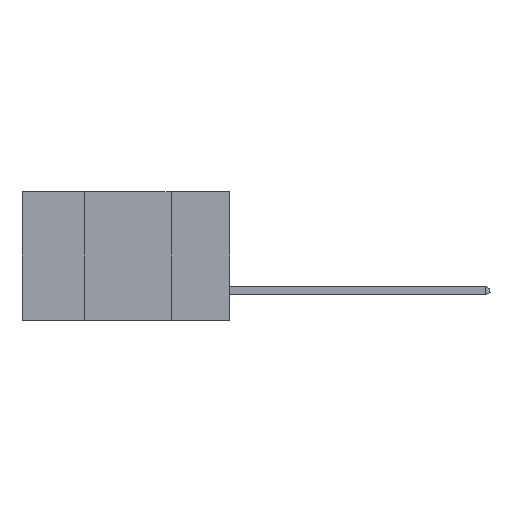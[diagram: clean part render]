
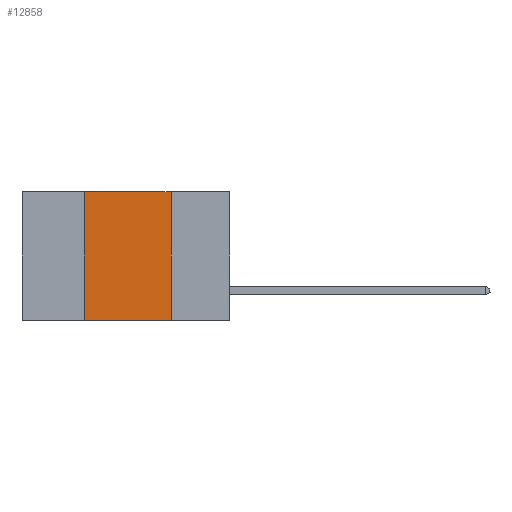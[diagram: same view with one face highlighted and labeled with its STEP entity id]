
A CAD part, left-side view. The second image highlights one B-rep face of the part: STEP entity #12858.
In plain terms, the highlighted planar face has unit normal (-1, 0, 0).
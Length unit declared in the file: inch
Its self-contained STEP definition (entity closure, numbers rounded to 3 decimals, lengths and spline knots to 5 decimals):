
#839 = DIRECTION ( 'NONE',  ( 0., -1., 0. ) ) ;
#905 = CARTESIAN_POINT ( 'NONE',  ( 0., 0.6, 0. ) ) ;
#2032 = ORIENTED_EDGE ( 'NONE', *, *, #14928, .F. ) ;
#2199 = PLANE ( 'NONE',  #7078 ) ;
#3323 = EDGE_CURVE ( 'NONE', #12522, #13117, #18465, .T. ) ;
#3673 = CARTESIAN_POINT ( 'NONE',  ( 0., 0.6, 0. ) ) ;
#4449 = CARTESIAN_POINT ( 'NONE',  ( 0., 0.17, -0.37 ) ) ;
#5538 = CARTESIAN_POINT ( 'NONE',  ( 0., 0.6, -0.37 ) ) ;
#5587 = ORIENTED_EDGE ( 'NONE', *, *, #17632, .T. ) ;
#5838 = LINE ( 'NONE', #13559, #14731 ) ;
#5912 = CARTESIAN_POINT ( 'NONE',  ( 0., 0.17, 0. ) ) ;
#6143 = CARTESIAN_POINT ( 'NONE',  ( 0., 0.42, 0. ) ) ;
#6190 = VECTOR ( 'NONE', #11976, 39.37008 ) ;
#6792 = VERTEX_POINT ( 'NONE', #4449 ) ;
#6851 = DIRECTION ( 'NONE',  ( 1., 0., 0. ) ) ;
#7078 = AXIS2_PLACEMENT_3D ( 'NONE', #3673, #6851, #8449 ) ;
#7102 = VERTEX_POINT ( 'NONE', #17599 ) ;
#7631 = EDGE_CURVE ( 'NONE', #7102, #12522, #5838, .T. ) ;
#8449 = DIRECTION ( 'NONE',  ( 0., 0., -1. ) ) ;
#9026 = ORIENTED_EDGE ( 'NONE', *, *, #3323, .F. ) ;
#9515 = VECTOR ( 'NONE', #10871, 39.37008 ) ;
#9770 = LINE ( 'NONE', #20231, #9515 ) ;
#10871 = DIRECTION ( 'NONE',  ( 0., 0., -1. ) ) ;
#11976 = DIRECTION ( 'NONE',  ( 0., -1., 0. ) ) ;
#12522 = VERTEX_POINT ( 'NONE', #6143 ) ;
#12666 = EDGE_LOOP ( 'NONE', ( #2032, #9026, #20257, #5587 ) ) ;
#12858 = ADVANCED_FACE ( 'NONE', ( #15710 ), #2199, .F. ) ;
#13117 = VERTEX_POINT ( 'NONE', #5912 ) ;
#13559 = CARTESIAN_POINT ( 'NONE',  ( 0., 0.42, 0. ) ) ;
#14731 = VECTOR ( 'NONE', #18426, 39.37008 ) ;
#14928 = EDGE_CURVE ( 'NONE', #13117, #6792, #9770, .T. ) ;
#15710 = FACE_OUTER_BOUND ( 'NONE', #12666, .T. ) ;
#17599 = CARTESIAN_POINT ( 'NONE',  ( 0., 0.42, -0.37 ) ) ;
#17632 = EDGE_CURVE ( 'NONE', #7102, #6792, #18735, .T. ) ;
#18236 = VECTOR ( 'NONE', #839, 39.37008 ) ;
#18426 = DIRECTION ( 'NONE',  ( 0., 0., 1. ) ) ;
#18465 = LINE ( 'NONE', #905, #18236 ) ;
#18735 = LINE ( 'NONE', #5538, #6190 ) ;
#20231 = CARTESIAN_POINT ( 'NONE',  ( 0., 0.17, 0. ) ) ;
#20257 = ORIENTED_EDGE ( 'NONE', *, *, #7631, .F. ) ;
